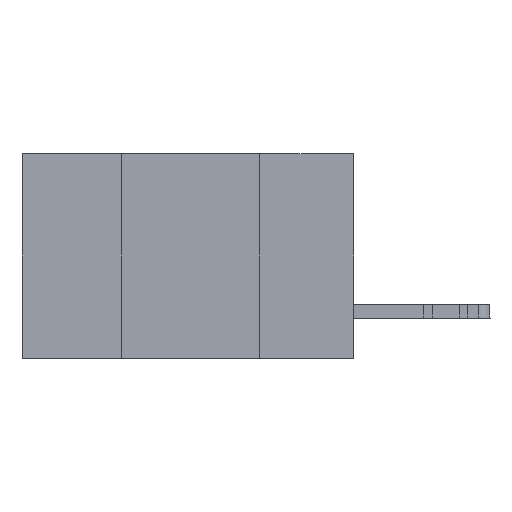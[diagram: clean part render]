
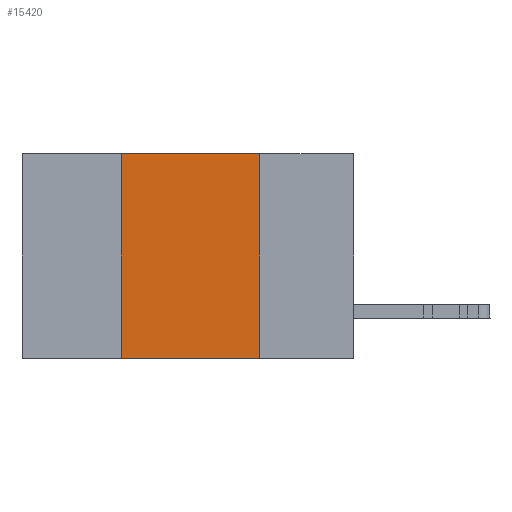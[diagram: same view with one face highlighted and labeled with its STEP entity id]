
A CAD part, left-side view. The second image highlights one B-rep face of the part: STEP entity #15420.
In plain terms, the highlighted planar face has unit normal (-1, 0, 0).
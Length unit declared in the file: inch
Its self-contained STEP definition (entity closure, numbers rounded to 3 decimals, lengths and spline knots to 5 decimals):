
#1026 = ORIENTED_EDGE ( 'NONE', *, *, #6827, .T. ) ;
#2334 = VERTEX_POINT ( 'NONE', #28116 ) ;
#2452 = VECTOR ( 'NONE', #47407, 39.37008 ) ;
#2460 = EDGE_LOOP ( 'NONE', ( #33075, #28173, #41157, #1026 ) ) ;
#3174 = VECTOR ( 'NONE', #4403, 39.37008 ) ;
#3883 = AXIS2_PLACEMENT_3D ( 'NONE', #6381, #6711, #13893 ) ;
#4403 = DIRECTION ( 'NONE',  ( 0., 0., 1. ) ) ;
#6163 = EDGE_CURVE ( 'NONE', #28842, #2334, #22316, .T. ) ;
#6381 = CARTESIAN_POINT ( 'NONE',  ( 0., 0.6, 0. ) ) ;
#6711 = DIRECTION ( 'NONE',  ( 1., 0., 0. ) ) ;
#6827 = EDGE_CURVE ( 'NONE', #28607, #36620, #27558, .T. ) ;
#8238 = DIRECTION ( 'NONE',  ( 0., -1., 0. ) ) ;
#9989 = CARTESIAN_POINT ( 'NONE',  ( 0., 0.6, 0. ) ) ;
#10861 = VECTOR ( 'NONE', #41580, 39.37008 ) ;
#12393 = EDGE_CURVE ( 'NONE', #28607, #28842, #13044, .T. ) ;
#13044 = LINE ( 'NONE', #30014, #3174 ) ;
#13893 = DIRECTION ( 'NONE',  ( 0., 0., -1. ) ) ;
#15420 = ADVANCED_FACE ( 'NONE', ( #29301 ), #32103, .F. ) ;
#17621 = VECTOR ( 'NONE', #8238, 39.37008 ) ;
#20210 = CARTESIAN_POINT ( 'NONE',  ( 0., 0.42, -0.37 ) ) ;
#22316 = LINE ( 'NONE', #9989, #2452 ) ;
#26453 = CARTESIAN_POINT ( 'NONE',  ( 0., 0.6, -0.37 ) ) ;
#27558 = LINE ( 'NONE', #26453, #17621 ) ;
#28116 = CARTESIAN_POINT ( 'NONE',  ( 0., 0.17, 0. ) ) ;
#28173 = ORIENTED_EDGE ( 'NONE', *, *, #6163, .F. ) ;
#28607 = VERTEX_POINT ( 'NONE', #20210 ) ;
#28842 = VERTEX_POINT ( 'NONE', #35830 ) ;
#29301 = FACE_OUTER_BOUND ( 'NONE', #2460, .T. ) ;
#30014 = CARTESIAN_POINT ( 'NONE',  ( 0., 0.42, 0. ) ) ;
#31973 = LINE ( 'NONE', #38309, #10861 ) ;
#32103 = PLANE ( 'NONE',  #3883 ) ;
#33075 = ORIENTED_EDGE ( 'NONE', *, *, #42634, .F. ) ;
#35830 = CARTESIAN_POINT ( 'NONE',  ( 0., 0.42, 0. ) ) ;
#36620 = VERTEX_POINT ( 'NONE', #47341 ) ;
#38309 = CARTESIAN_POINT ( 'NONE',  ( 0., 0.17, 0. ) ) ;
#41157 = ORIENTED_EDGE ( 'NONE', *, *, #12393, .F. ) ;
#41580 = DIRECTION ( 'NONE',  ( 0., 0., -1. ) ) ;
#42634 = EDGE_CURVE ( 'NONE', #2334, #36620, #31973, .T. ) ;
#47341 = CARTESIAN_POINT ( 'NONE',  ( 0., 0.17, -0.37 ) ) ;
#47407 = DIRECTION ( 'NONE',  ( 0., -1., 0. ) ) ;
